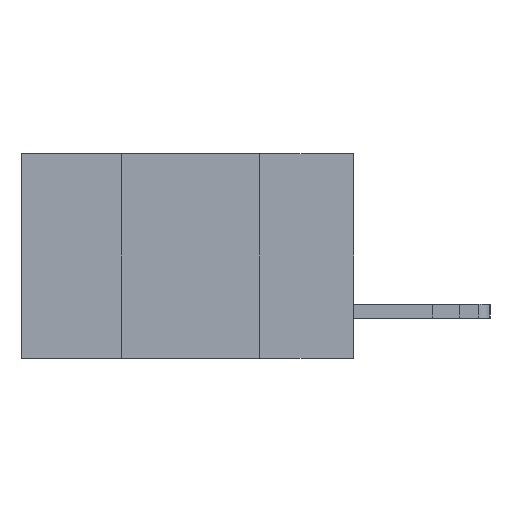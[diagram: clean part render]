
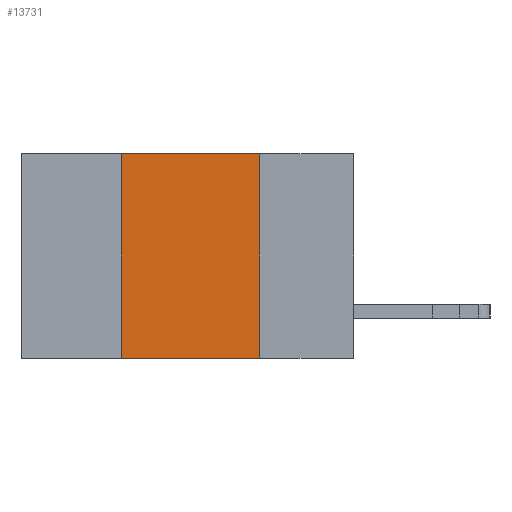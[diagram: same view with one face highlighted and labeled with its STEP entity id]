
A CAD part, left-side view. The second image highlights one B-rep face of the part: STEP entity #13731.
In plain terms, the highlighted planar face has unit normal (-1, 0, 0).
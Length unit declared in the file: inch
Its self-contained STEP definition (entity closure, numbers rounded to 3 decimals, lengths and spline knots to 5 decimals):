
#761 = VERTEX_POINT ( 'NONE', #1457 ) ;
#1137 = ORIENTED_EDGE ( 'NONE', *, *, #10034, .T. ) ;
#1158 = VECTOR ( 'NONE', #14461, 39.37008 ) ;
#1370 = VERTEX_POINT ( 'NONE', #15081 ) ;
#1457 = CARTESIAN_POINT ( 'NONE',  ( 0., 0.42, -0.37 ) ) ;
#2035 = CARTESIAN_POINT ( 'NONE',  ( 0., 0.17, 0. ) ) ;
#2240 = EDGE_CURVE ( 'NONE', #5533, #1370, #8179, .T. ) ;
#2678 = CARTESIAN_POINT ( 'NONE',  ( 0., 0.6, -0.37 ) ) ;
#3440 = DIRECTION ( 'NONE',  ( 0., 0., -1. ) ) ;
#3546 = EDGE_LOOP ( 'NONE', ( #8947, #14044, #7896, #1137 ) ) ;
#3577 = CARTESIAN_POINT ( 'NONE',  ( 0., 0.17, 0. ) ) ;
#3603 = DIRECTION ( 'NONE',  ( 1., 0., 0. ) ) ;
#3977 = VECTOR ( 'NONE', #8125, 39.37008 ) ;
#5322 = VECTOR ( 'NONE', #12815, 39.37008 ) ;
#5533 = VERTEX_POINT ( 'NONE', #3577 ) ;
#7896 = ORIENTED_EDGE ( 'NONE', *, *, #10954, .F. ) ;
#8125 = DIRECTION ( 'NONE',  ( 0., 0., 1. ) ) ;
#8179 = LINE ( 'NONE', #2035, #12705 ) ;
#8245 = CARTESIAN_POINT ( 'NONE',  ( 0., 0.6, 0. ) ) ;
#8408 = DIRECTION ( 'NONE',  ( 0., 0., -1. ) ) ;
#8947 = ORIENTED_EDGE ( 'NONE', *, *, #2240, .F. ) ;
#9258 = LINE ( 'NONE', #10582, #3977 ) ;
#9490 = FACE_OUTER_BOUND ( 'NONE', #3546, .T. ) ;
#9729 = PLANE ( 'NONE',  #13191 ) ;
#10034 = EDGE_CURVE ( 'NONE', #761, #1370, #13807, .T. ) ;
#10582 = CARTESIAN_POINT ( 'NONE',  ( 0., 0.42, 0. ) ) ;
#10946 = LINE ( 'NONE', #8245, #1158 ) ;
#10954 = EDGE_CURVE ( 'NONE', #761, #12235, #9258, .T. ) ;
#12235 = VERTEX_POINT ( 'NONE', #12402 ) ;
#12402 = CARTESIAN_POINT ( 'NONE',  ( 0., 0.42, 0. ) ) ;
#12705 = VECTOR ( 'NONE', #8408, 39.37008 ) ;
#12815 = DIRECTION ( 'NONE',  ( 0., -1., 0. ) ) ;
#12966 = EDGE_CURVE ( 'NONE', #12235, #5533, #10946, .T. ) ;
#13191 = AXIS2_PLACEMENT_3D ( 'NONE', #14568, #3603, #3440 ) ;
#13731 = ADVANCED_FACE ( 'NONE', ( #9490 ), #9729, .F. ) ;
#13807 = LINE ( 'NONE', #2678, #5322 ) ;
#14044 = ORIENTED_EDGE ( 'NONE', *, *, #12966, .F. ) ;
#14461 = DIRECTION ( 'NONE',  ( 0., -1., 0. ) ) ;
#14568 = CARTESIAN_POINT ( 'NONE',  ( 0., 0.6, 0. ) ) ;
#15081 = CARTESIAN_POINT ( 'NONE',  ( 0., 0.17, -0.37 ) ) ;
